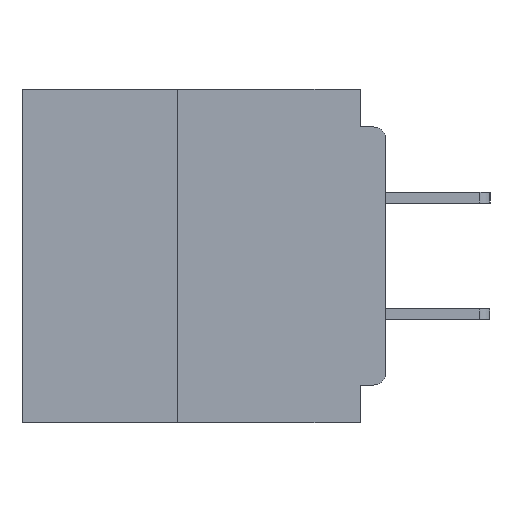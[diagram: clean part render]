
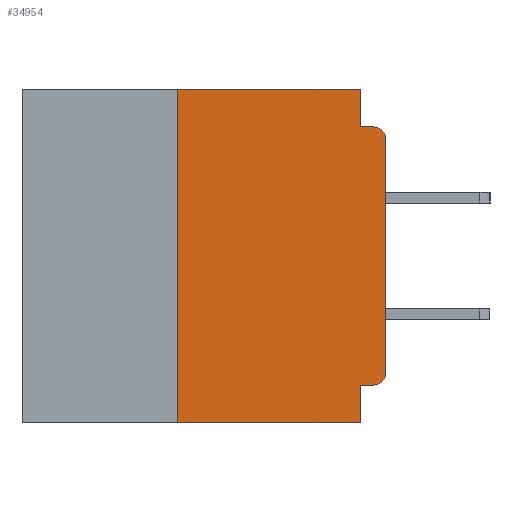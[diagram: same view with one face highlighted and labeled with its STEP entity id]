
A CAD part, left-side view. The second image highlights one B-rep face of the part: STEP entity #34954.
In plain terms, the highlighted planar face has unit normal (-1, 0, 0).
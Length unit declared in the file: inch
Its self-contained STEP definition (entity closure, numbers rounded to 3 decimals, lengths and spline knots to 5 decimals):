
#428 = CIRCLE ( 'NONE', #43943, 0.015 ) ;
#701 = CARTESIAN_POINT ( 'NONE',  ( 0., 0.031, -0.355 ) ) ;
#1115 = CARTESIAN_POINT ( 'NONE',  ( 0., 0.015, -0.34 ) ) ;
#2530 = LINE ( 'NONE', #25014, #38609 ) ;
#2547 = ORIENTED_EDGE ( 'NONE', *, *, #29343, .T. ) ;
#2602 = VERTEX_POINT ( 'NONE', #12117 ) ;
#3181 = DIRECTION ( 'NONE',  ( -1., 0., 0. ) ) ;
#4285 = DIRECTION ( 'NONE',  ( 0., -1., 0. ) ) ;
#5686 = DIRECTION ( 'NONE',  ( 0., 0., -1. ) ) ;
#6050 = AXIS2_PLACEMENT_3D ( 'NONE', #30303, #3181, #34860 ) ;
#7404 = EDGE_CURVE ( 'NONE', #11293, #11532, #7799, .T. ) ;
#7585 = VERTEX_POINT ( 'NONE', #42150 ) ;
#7799 = LINE ( 'NONE', #40823, #36786 ) ;
#7914 = VECTOR ( 'NONE', #4285, 39.37008 ) ;
#7935 = EDGE_LOOP ( 'NONE', ( #43828, #2547, #40958, #45058, #23966, #33676, #10452, #26724, #48069, #31556 ) ) ;
#10452 = ORIENTED_EDGE ( 'NONE', *, *, #28313, .T. ) ;
#11293 = VERTEX_POINT ( 'NONE', #30854 ) ;
#11532 = VERTEX_POINT ( 'NONE', #701 ) ;
#12117 = CARTESIAN_POINT ( 'NONE',  ( 0., 0.031, 0. ) ) ;
#12392 = EDGE_CURVE ( 'NONE', #18629, #2602, #2530, .T. ) ;
#12439 = EDGE_CURVE ( 'NONE', #2602, #34190, #50535, .T. ) ;
#12762 = AXIS2_PLACEMENT_3D ( 'NONE', #27160, #21690, #31672 ) ;
#12841 = VERTEX_POINT ( 'NONE', #42475 ) ;
#12929 = VECTOR ( 'NONE', #53885, 39.37008 ) ;
#13296 = CARTESIAN_POINT ( 'NONE',  ( 0., 0., 0. ) ) ;
#14675 = CIRCLE ( 'NONE', #6050, 0.015 ) ;
#15924 = DIRECTION ( 'NONE',  ( 0., -1., 0. ) ) ;
#16374 = LINE ( 'NONE', #28261, #38942 ) ;
#16986 = CARTESIAN_POINT ( 'NONE',  ( 0., 0.25, -0.4 ) ) ;
#18629 = VERTEX_POINT ( 'NONE', #51675 ) ;
#19745 = EDGE_CURVE ( 'NONE', #11532, #20559, #16374, .T. ) ;
#20559 = VERTEX_POINT ( 'NONE', #33910 ) ;
#21329 = LINE ( 'NONE', #16986, #54363 ) ;
#21690 = DIRECTION ( 'NONE',  ( 1., 0., 0. ) ) ;
#22177 = VECTOR ( 'NONE', #43889, 39.37008 ) ;
#22877 = CARTESIAN_POINT ( 'NONE',  ( 0., 0.015, -0.045 ) ) ;
#23966 = ORIENTED_EDGE ( 'NONE', *, *, #12392, .F. ) ;
#25014 = CARTESIAN_POINT ( 'NONE',  ( 0., 0.437, 0. ) ) ;
#25969 = CARTESIAN_POINT ( 'NONE',  ( 0., 0., -0.045 ) ) ;
#26724 = ORIENTED_EDGE ( 'NONE', *, *, #19745, .F. ) ;
#27119 = VERTEX_POINT ( 'NONE', #45540 ) ;
#27160 = CARTESIAN_POINT ( 'NONE',  ( 0., 0.437, 0. ) ) ;
#27683 = VERTEX_POINT ( 'NONE', #22877 ) ;
#28261 = CARTESIAN_POINT ( 'NONE',  ( 0., 0.031, -0.4 ) ) ;
#28313 = EDGE_CURVE ( 'NONE', #7585, #20559, #55834, .T. ) ;
#29343 = EDGE_CURVE ( 'NONE', #27119, #27683, #14675, .T. ) ;
#29942 = DIRECTION ( 'NONE',  ( 0., 0., -1. ) ) ;
#30303 = CARTESIAN_POINT ( 'NONE',  ( 0., 0.015, -0.06 ) ) ;
#30854 = CARTESIAN_POINT ( 'NONE',  ( 0., 0.015, -0.355 ) ) ;
#31556 = ORIENTED_EDGE ( 'NONE', *, *, #39779, .T. ) ;
#31672 = DIRECTION ( 'NONE',  ( 0., 0., -1. ) ) ;
#32699 = EDGE_CURVE ( 'NONE', #34190, #27683, #46093, .T. ) ;
#32808 = DIRECTION ( 'NONE',  ( -1., 0., 0. ) ) ;
#33676 = ORIENTED_EDGE ( 'NONE', *, *, #45436, .F. ) ;
#33910 = CARTESIAN_POINT ( 'NONE',  ( 0., 0.031, -0.4 ) ) ;
#34190 = VERTEX_POINT ( 'NONE', #39444 ) ;
#34397 = VECTOR ( 'NONE', #29942, 39.37008 ) ;
#34860 = DIRECTION ( 'NONE',  ( 0., 0., -1. ) ) ;
#34954 = ADVANCED_FACE ( 'NONE', ( #57749 ), #54059, .F. ) ;
#35933 = CARTESIAN_POINT ( 'NONE',  ( 0., 0.437, -0.4 ) ) ;
#36786 = VECTOR ( 'NONE', #45325, 39.37008 ) ;
#38609 = VECTOR ( 'NONE', #15924, 39.37008 ) ;
#38942 = VECTOR ( 'NONE', #55147, 39.37008 ) ;
#39444 = CARTESIAN_POINT ( 'NONE',  ( 0., 0.031, -0.045 ) ) ;
#39779 = EDGE_CURVE ( 'NONE', #11293, #12841, #428, .T. ) ;
#39801 = LINE ( 'NONE', #13296, #12929 ) ;
#40823 = CARTESIAN_POINT ( 'NONE',  ( 0., 0., -0.355 ) ) ;
#40958 = ORIENTED_EDGE ( 'NONE', *, *, #32699, .F. ) ;
#42150 = CARTESIAN_POINT ( 'NONE',  ( 0., 0.25, -0.4 ) ) ;
#42475 = CARTESIAN_POINT ( 'NONE',  ( 0., 0., -0.34 ) ) ;
#43315 = CARTESIAN_POINT ( 'NONE',  ( 0., 0.031, 0. ) ) ;
#43828 = ORIENTED_EDGE ( 'NONE', *, *, #44298, .T. ) ;
#43889 = DIRECTION ( 'NONE',  ( 0., -1., 0. ) ) ;
#43943 = AXIS2_PLACEMENT_3D ( 'NONE', #1115, #32808, #5686 ) ;
#44298 = EDGE_CURVE ( 'NONE', #12841, #27119, #39801, .T. ) ;
#45058 = ORIENTED_EDGE ( 'NONE', *, *, #12439, .F. ) ;
#45325 = DIRECTION ( 'NONE',  ( 0., 1., 0. ) ) ;
#45436 = EDGE_CURVE ( 'NONE', #7585, #18629, #21329, .T. ) ;
#45540 = CARTESIAN_POINT ( 'NONE',  ( 0., 0., -0.06 ) ) ;
#46093 = LINE ( 'NONE', #25969, #22177 ) ;
#48069 = ORIENTED_EDGE ( 'NONE', *, *, #7404, .F. ) ;
#48312 = DIRECTION ( 'NONE',  ( 0., 0., 1. ) ) ;
#50535 = LINE ( 'NONE', #43315, #34397 ) ;
#51675 = CARTESIAN_POINT ( 'NONE',  ( 0., 0.25, 0. ) ) ;
#53885 = DIRECTION ( 'NONE',  ( 0., 0., 1. ) ) ;
#54059 = PLANE ( 'NONE',  #12762 ) ;
#54363 = VECTOR ( 'NONE', #48312, 39.37008 ) ;
#55147 = DIRECTION ( 'NONE',  ( 0., 0., -1. ) ) ;
#55834 = LINE ( 'NONE', #35933, #7914 ) ;
#57749 = FACE_OUTER_BOUND ( 'NONE', #7935, .T. ) ;
